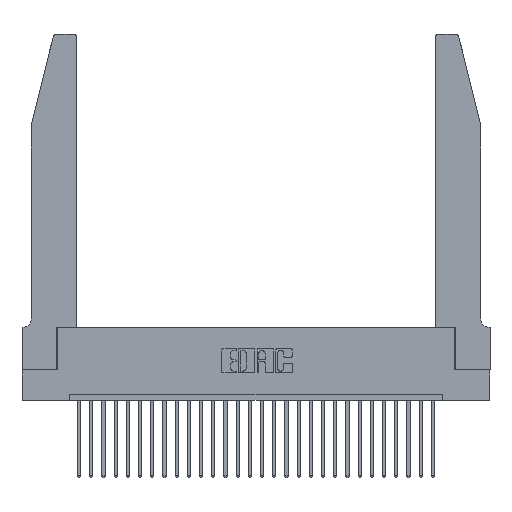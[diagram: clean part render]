
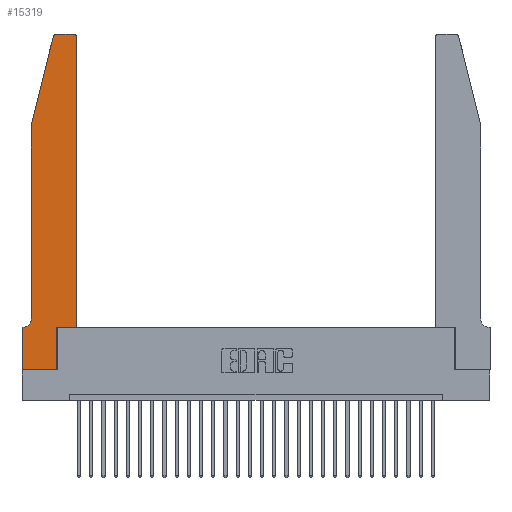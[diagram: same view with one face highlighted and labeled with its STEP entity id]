
A CAD part, top view. The second image highlights one B-rep face of the part: STEP entity #15319.
In plain terms, the highlighted planar face has unit normal (0, 0, 1).
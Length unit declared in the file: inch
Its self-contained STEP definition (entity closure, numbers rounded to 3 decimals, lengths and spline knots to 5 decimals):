
#398 = AXIS2_PLACEMENT_3D ( 'NONE', #2229, #20508, #26783 ) ;
#679 = VERTEX_POINT ( 'NONE', #15820 ) ;
#1536 = CARTESIAN_POINT ( 'NONE',  ( 0., 0., 0.37 ) ) ;
#1569 = CARTESIAN_POINT ( 'NONE',  ( 0., 0., 0.37 ) ) ;
#1598 = DIRECTION ( 'NONE',  ( -1., 0., 0. ) ) ;
#1834 = VERTEX_POINT ( 'NONE', #14738 ) ;
#2033 = DIRECTION ( 'NONE',  ( -1., 0., 0. ) ) ;
#2169 = EDGE_CURVE ( 'NONE', #5791, #2176, #13884, .T. ) ;
#2176 = VERTEX_POINT ( 'NONE', #24806 ) ;
#2229 = CARTESIAN_POINT ( 'NONE',  ( 0.0055, 0.42, 0.37 ) ) ;
#2409 = CARTESIAN_POINT ( 'NONE',  ( 0.2865, 0.35, 0.37 ) ) ;
#2825 = CARTESIAN_POINT ( 'NONE',  ( 0.0755, 2., 0.37 ) ) ;
#2911 = ORIENTED_EDGE ( 'NONE', *, *, #3153, .T. ) ;
#2994 = DIRECTION ( 'NONE',  ( 1., 0., 0. ) ) ;
#3153 = EDGE_CURVE ( 'NONE', #15100, #5791, #8579, .T. ) ;
#3177 = ORIENTED_EDGE ( 'NONE', *, *, #4123, .T. ) ;
#3264 = PLANE ( 'NONE',  #12602 ) ;
#3408 = VECTOR ( 'NONE', #8865, 39.37008 ) ;
#3661 = CARTESIAN_POINT ( 'NONE',  ( 0.4205, 2.75, 0.37 ) ) ;
#3671 = EDGE_CURVE ( 'NONE', #23168, #15281, #15420, .T. ) ;
#4123 = EDGE_CURVE ( 'NONE', #5536, #23168, #5545, .T. ) ;
#4174 = ORIENTED_EDGE ( 'NONE', *, *, #14776, .T. ) ;
#4397 = VECTOR ( 'NONE', #6888, 39.37008 ) ;
#4539 = EDGE_CURVE ( 'NONE', #8405, #1834, #16074, .T. ) ;
#5170 = VECTOR ( 'NONE', #7470, 39.37008 ) ;
#5238 = LINE ( 'NONE', #13943, #7325 ) ;
#5250 = CARTESIAN_POINT ( 'NONE',  ( 0.4205, 2.72, 0.37 ) ) ;
#5505 = CARTESIAN_POINT ( 'NONE',  ( 0., 0.35, 0.37 ) ) ;
#5536 = VERTEX_POINT ( 'NONE', #3661 ) ;
#5545 = LINE ( 'NONE', #24162, #7648 ) ;
#5708 = EDGE_CURVE ( 'NONE', #21060, #15100, #19877, .T. ) ;
#5791 = VERTEX_POINT ( 'NONE', #15652 ) ;
#6376 = CIRCLE ( 'NONE', #25263, 0.03 ) ;
#6547 = DIRECTION ( 'NONE',  ( 0., 0., 1. ) ) ;
#6796 = DIRECTION ( 'NONE',  ( 0., 1., 0. ) ) ;
#6888 = DIRECTION ( 'NONE',  ( -0.239, -0.971, 0. ) ) ;
#7325 = VECTOR ( 'NONE', #2994, 39.37008 ) ;
#7470 = DIRECTION ( 'NONE',  ( 0., -1., 0. ) ) ;
#7648 = VECTOR ( 'NONE', #2033, 39.37008 ) ;
#8044 = VERTEX_POINT ( 'NONE', #20861 ) ;
#8141 = ORIENTED_EDGE ( 'NONE', *, *, #21966, .T. ) ;
#8405 = VERTEX_POINT ( 'NONE', #17922 ) ;
#8579 = LINE ( 'NONE', #1536, #13817 ) ;
#8586 = CARTESIAN_POINT ( 'NONE',  ( 0., 0., 0.37 ) ) ;
#8865 = DIRECTION ( 'NONE',  ( 0., -1., 0. ) ) ;
#10126 = VERTEX_POINT ( 'NONE', #16195 ) ;
#10273 = ORIENTED_EDGE ( 'NONE', *, *, #22158, .T. ) ;
#10781 = EDGE_CURVE ( 'NONE', #10126, #21060, #11303, .T. ) ;
#10959 = ORIENTED_EDGE ( 'NONE', *, *, #2169, .T. ) ;
#11303 = LINE ( 'NONE', #15036, #28428 ) ;
#11984 = EDGE_LOOP ( 'NONE', ( #3177, #15761, #4174, #15590, #8141, #28890, #25024, #2911, #10959, #10273, #12001, #19418 ) ) ;
#11990 = VECTOR ( 'NONE', #6796, 39.37008 ) ;
#12001 = ORIENTED_EDGE ( 'NONE', *, *, #25744, .T. ) ;
#12602 = AXIS2_PLACEMENT_3D ( 'NONE', #5505, #21292, #23446 ) ;
#12612 = DIRECTION ( 'NONE',  ( 1., 0., 0. ) ) ;
#13244 = CARTESIAN_POINT ( 'NONE',  ( 0., 0.35, 0.37 ) ) ;
#13516 = FACE_OUTER_BOUND ( 'NONE', #11984, .T. ) ;
#13817 = VECTOR ( 'NONE', #19233, 39.37008 ) ;
#13828 = DIRECTION ( 'NONE',  ( 0., 1., 0. ) ) ;
#13884 = LINE ( 'NONE', #2409, #28915 ) ;
#13943 = CARTESIAN_POINT ( 'NONE',  ( 0.4505, 0.35, 0.37 ) ) ;
#14738 = CARTESIAN_POINT ( 'NONE',  ( 0.0755, 0.42, 0.37 ) ) ;
#14776 = EDGE_CURVE ( 'NONE', #15281, #8405, #20166, .T. ) ;
#15036 = CARTESIAN_POINT ( 'NONE',  ( 0.0755, 0.35, 0.37 ) ) ;
#15100 = VERTEX_POINT ( 'NONE', #1569 ) ;
#15281 = VERTEX_POINT ( 'NONE', #21483 ) ;
#15319 = ADVANCED_FACE ( 'NONE', ( #13516 ), #3264, .T. ) ;
#15420 = CIRCLE ( 'NONE', #24961, 0.03 ) ;
#15493 = CARTESIAN_POINT ( 'NONE',  ( 0.4505, 0.35, 0.37 ) ) ;
#15590 = ORIENTED_EDGE ( 'NONE', *, *, #4539, .T. ) ;
#15652 = CARTESIAN_POINT ( 'NONE',  ( 0.2865, 0., 0.37 ) ) ;
#15761 = ORIENTED_EDGE ( 'NONE', *, *, #3671, .T. ) ;
#15820 = CARTESIAN_POINT ( 'NONE',  ( 0.4505, 2.72, 0.37 ) ) ;
#16074 = LINE ( 'NONE', #2825, #5170 ) ;
#16195 = CARTESIAN_POINT ( 'NONE',  ( 0.0055, 0.35, 0.37 ) ) ;
#16552 = DIRECTION ( 'NONE',  ( 0., 0., 1. ) ) ;
#17922 = CARTESIAN_POINT ( 'NONE',  ( 0.0755, 2., 0.37 ) ) ;
#17928 = LINE ( 'NONE', #15493, #11990 ) ;
#17984 = CARTESIAN_POINT ( 'NONE',  ( 0.0755, 2., 0.37 ) ) ;
#19233 = DIRECTION ( 'NONE',  ( 1., 0., 0. ) ) ;
#19418 = ORIENTED_EDGE ( 'NONE', *, *, #19745, .T. ) ;
#19745 = EDGE_CURVE ( 'NONE', #679, #5536, #6376, .T. ) ;
#19877 = LINE ( 'NONE', #8586, #3408 ) ;
#20166 = LINE ( 'NONE', #17984, #4397 ) ;
#20508 = DIRECTION ( 'NONE',  ( 0., 0., -1. ) ) ;
#20861 = CARTESIAN_POINT ( 'NONE',  ( 0.4505, 0.35, 0.37 ) ) ;
#21060 = VERTEX_POINT ( 'NONE', #13244 ) ;
#21292 = DIRECTION ( 'NONE',  ( 0., 0., 1. ) ) ;
#21483 = CARTESIAN_POINT ( 'NONE',  ( 0.25487, 2.72718, 0.37 ) ) ;
#21754 = CIRCLE ( 'NONE', #398, 0.07 ) ;
#21966 = EDGE_CURVE ( 'NONE', #1834, #10126, #21754, .T. ) ;
#22158 = EDGE_CURVE ( 'NONE', #2176, #8044, #5238, .T. ) ;
#22539 = CARTESIAN_POINT ( 'NONE',  ( 0.284, 2.72, 0.37 ) ) ;
#22636 = DIRECTION ( 'NONE',  ( 1., 0., 0. ) ) ;
#23168 = VERTEX_POINT ( 'NONE', #24010 ) ;
#23446 = DIRECTION ( 'NONE',  ( 1., 0., 0. ) ) ;
#24010 = CARTESIAN_POINT ( 'NONE',  ( 0.284, 2.75, 0.37 ) ) ;
#24162 = CARTESIAN_POINT ( 'NONE',  ( 0.2605, 2.75, 0.37 ) ) ;
#24806 = CARTESIAN_POINT ( 'NONE',  ( 0.2865, 0.35, 0.37 ) ) ;
#24961 = AXIS2_PLACEMENT_3D ( 'NONE', #22539, #6547, #22636 ) ;
#25024 = ORIENTED_EDGE ( 'NONE', *, *, #5708, .T. ) ;
#25263 = AXIS2_PLACEMENT_3D ( 'NONE', #5250, #16552, #12612 ) ;
#25744 = EDGE_CURVE ( 'NONE', #8044, #679, #17928, .T. ) ;
#26783 = DIRECTION ( 'NONE',  ( -1., 0., 0. ) ) ;
#28428 = VECTOR ( 'NONE', #1598, 39.37008 ) ;
#28890 = ORIENTED_EDGE ( 'NONE', *, *, #10781, .T. ) ;
#28915 = VECTOR ( 'NONE', #13828, 39.37008 ) ;
